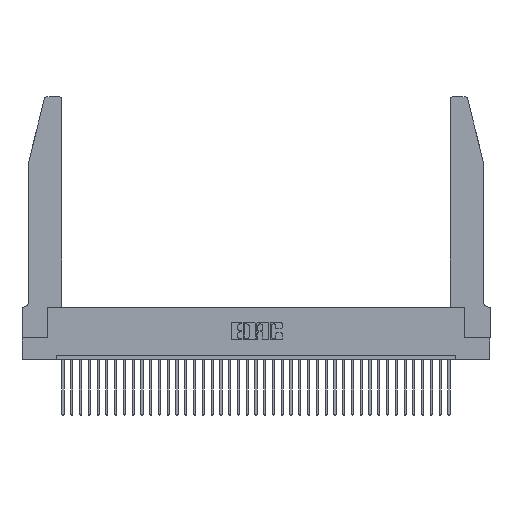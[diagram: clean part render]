
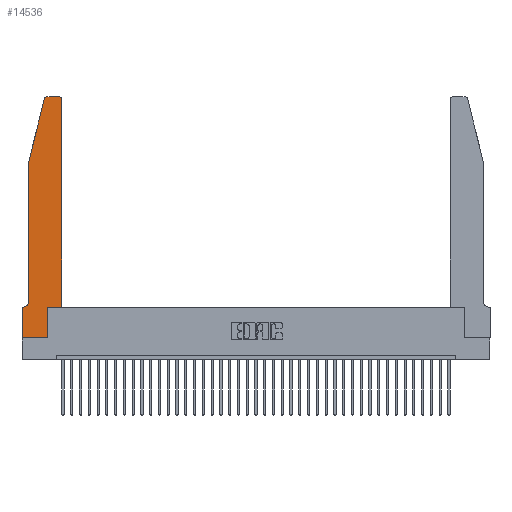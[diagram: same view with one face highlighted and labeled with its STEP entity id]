
A CAD part, top view. The second image highlights one B-rep face of the part: STEP entity #14536.
In plain terms, the highlighted planar face has unit normal (0, 0, 1).
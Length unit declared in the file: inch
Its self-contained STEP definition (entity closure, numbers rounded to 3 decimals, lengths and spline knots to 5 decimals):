
#27 = ORIENTED_EDGE ( 'NONE', *, *, #2586, .T. ) ;
#439 = VERTEX_POINT ( 'NONE', #1338 ) ;
#661 = LINE ( 'NONE', #3811, #19276 ) ;
#669 = DIRECTION ( 'NONE',  ( 1., 0., 0. ) ) ;
#900 = ORIENTED_EDGE ( 'NONE', *, *, #21113, .T. ) ;
#1338 = CARTESIAN_POINT ( 'NONE',  ( 0.284, 2.75, 0.37 ) ) ;
#1552 = ORIENTED_EDGE ( 'NONE', *, *, #27397, .T. ) ;
#1887 = EDGE_CURVE ( 'NONE', #439, #12241, #6059, .T. ) ;
#2379 = DIRECTION ( 'NONE',  ( 1., 0., 0. ) ) ;
#2560 = VECTOR ( 'NONE', #28213, 39.37008 ) ;
#2586 = EDGE_CURVE ( 'NONE', #36108, #38092, #12020, .T. ) ;
#3017 = VECTOR ( 'NONE', #18549, 39.37008 ) ;
#3510 = ORIENTED_EDGE ( 'NONE', *, *, #21230, .T. ) ;
#3811 = CARTESIAN_POINT ( 'NONE',  ( 0.4505, 0.35, 0.37 ) ) ;
#4229 = DIRECTION ( 'NONE',  ( 0., -1., 0. ) ) ;
#4779 = CARTESIAN_POINT ( 'NONE',  ( 0., 0., 0.37 ) ) ;
#5054 = EDGE_CURVE ( 'NONE', #34523, #29858, #28505, .T. ) ;
#5510 = ORIENTED_EDGE ( 'NONE', *, *, #1887, .T. ) ;
#5737 = AXIS2_PLACEMENT_3D ( 'NONE', #20176, #38187, #2379 ) ;
#6059 = CIRCLE ( 'NONE', #23734, 0.03 ) ;
#6808 = CARTESIAN_POINT ( 'NONE',  ( 0.4505, 0.35, 0.37 ) ) ;
#7506 = CARTESIAN_POINT ( 'NONE',  ( 0.4505, 2.72, 0.37 ) ) ;
#7575 = EDGE_CURVE ( 'NONE', #21696, #34523, #20828, .T. ) ;
#7749 = CARTESIAN_POINT ( 'NONE',  ( 0.4505, 0.35, 0.37 ) ) ;
#7900 = DIRECTION ( 'NONE',  ( 1., 0., 0. ) ) ;
#7916 = VERTEX_POINT ( 'NONE', #7506 ) ;
#8160 = DIRECTION ( 'NONE',  ( 1., 0., 0. ) ) ;
#8481 = CARTESIAN_POINT ( 'NONE',  ( 0.0055, 0.35, 0.37 ) ) ;
#9003 = DIRECTION ( 'NONE',  ( 0., 0., 1. ) ) ;
#9272 = LINE ( 'NONE', #36241, #23225 ) ;
#9923 = EDGE_CURVE ( 'NONE', #19234, #21696, #10571, .T. ) ;
#9963 = ORIENTED_EDGE ( 'NONE', *, *, #11675, .T. ) ;
#10032 = CARTESIAN_POINT ( 'NONE',  ( 0.2865, 0., 0.37 ) ) ;
#10311 = AXIS2_PLACEMENT_3D ( 'NONE', #26626, #9003, #669 ) ;
#10571 = LINE ( 'NONE', #36895, #30938 ) ;
#10976 = VERTEX_POINT ( 'NONE', #34652 ) ;
#11675 = EDGE_CURVE ( 'NONE', #7916, #10976, #25784, .T. ) ;
#11745 = VECTOR ( 'NONE', #31426, 39.37008 ) ;
#11916 = EDGE_CURVE ( 'NONE', #13918, #7916, #661, .T. ) ;
#12020 = LINE ( 'NONE', #12083, #21261 ) ;
#12083 = CARTESIAN_POINT ( 'NONE',  ( 0.2865, 0.35, 0.37 ) ) ;
#12241 = VERTEX_POINT ( 'NONE', #16559 ) ;
#12254 = LINE ( 'NONE', #35901, #3017 ) ;
#12958 = CARTESIAN_POINT ( 'NONE',  ( 0.2865, 0.35, 0.37 ) ) ;
#13741 = CARTESIAN_POINT ( 'NONE',  ( 0., 0., 0.37 ) ) ;
#13918 = VERTEX_POINT ( 'NONE', #6808 ) ;
#13944 = CARTESIAN_POINT ( 'NONE',  ( 0.0055, 0.42, 0.37 ) ) ;
#14076 = DIRECTION ( 'NONE',  ( 0., 0., -1. ) ) ;
#14536 = ADVANCED_FACE ( 'NONE', ( #22300 ), #17687, .T. ) ;
#14824 = EDGE_CURVE ( 'NONE', #10976, #439, #9272, .T. ) ;
#14946 = CARTESIAN_POINT ( 'NONE',  ( 0.284, 2.72, 0.37 ) ) ;
#15090 = DIRECTION ( 'NONE',  ( 0., 1., 0. ) ) ;
#16528 = ORIENTED_EDGE ( 'NONE', *, *, #7575, .T. ) ;
#16559 = CARTESIAN_POINT ( 'NONE',  ( 0.25487, 2.72718, 0.37 ) ) ;
#17304 = ORIENTED_EDGE ( 'NONE', *, *, #29961, .T. ) ;
#17687 = PLANE ( 'NONE',  #10311 ) ;
#18549 = DIRECTION ( 'NONE',  ( -0.239, -0.971, 0. ) ) ;
#19234 = VERTEX_POINT ( 'NONE', #24349 ) ;
#19276 = VECTOR ( 'NONE', #30880, 39.37008 ) ;
#20176 = CARTESIAN_POINT ( 'NONE',  ( 0.4205, 2.72, 0.37 ) ) ;
#20180 = VERTEX_POINT ( 'NONE', #24762 ) ;
#20828 = CIRCLE ( 'NONE', #27363, 0.07 ) ;
#21113 = EDGE_CURVE ( 'NONE', #20180, #36108, #26220, .T. ) ;
#21230 = EDGE_CURVE ( 'NONE', #12241, #19234, #12254, .T. ) ;
#21261 = VECTOR ( 'NONE', #15090, 39.37008 ) ;
#21696 = VERTEX_POINT ( 'NONE', #31129 ) ;
#22029 = LINE ( 'NONE', #7749, #2560 ) ;
#22300 = FACE_OUTER_BOUND ( 'NONE', #22738, .T. ) ;
#22738 = EDGE_LOOP ( 'NONE', ( #34555, #5510, #3510, #27097, #16528, #27089, #1552, #900, #27, #17304, #29518, #9963 ) ) ;
#23225 = VECTOR ( 'NONE', #33301, 39.37008 ) ;
#23734 = AXIS2_PLACEMENT_3D ( 'NONE', #14946, #23976, #8160 ) ;
#23976 = DIRECTION ( 'NONE',  ( 0., 0., 1. ) ) ;
#24349 = CARTESIAN_POINT ( 'NONE',  ( 0.0755, 2., 0.37 ) ) ;
#24762 = CARTESIAN_POINT ( 'NONE',  ( 0., 0., 0.37 ) ) ;
#25153 = DIRECTION ( 'NONE',  ( -1., 0., 0. ) ) ;
#25784 = CIRCLE ( 'NONE', #5737, 0.03 ) ;
#26220 = LINE ( 'NONE', #13741, #32194 ) ;
#26626 = CARTESIAN_POINT ( 'NONE',  ( 0., 0.35, 0.37 ) ) ;
#27050 = CARTESIAN_POINT ( 'NONE',  ( 0.0755, 0.35, 0.37 ) ) ;
#27089 = ORIENTED_EDGE ( 'NONE', *, *, #5054, .T. ) ;
#27097 = ORIENTED_EDGE ( 'NONE', *, *, #9923, .T. ) ;
#27363 = AXIS2_PLACEMENT_3D ( 'NONE', #13944, #14076, #32129 ) ;
#27397 = EDGE_CURVE ( 'NONE', #29858, #20180, #35291, .T. ) ;
#28213 = DIRECTION ( 'NONE',  ( 1., 0., 0. ) ) ;
#28474 = CARTESIAN_POINT ( 'NONE',  ( 0., 0.35, 0.37 ) ) ;
#28505 = LINE ( 'NONE', #27050, #29391 ) ;
#29391 = VECTOR ( 'NONE', #25153, 39.37008 ) ;
#29518 = ORIENTED_EDGE ( 'NONE', *, *, #11916, .T. ) ;
#29858 = VERTEX_POINT ( 'NONE', #28474 ) ;
#29961 = EDGE_CURVE ( 'NONE', #38092, #13918, #22029, .T. ) ;
#30880 = DIRECTION ( 'NONE',  ( 0., 1., 0. ) ) ;
#30938 = VECTOR ( 'NONE', #4229, 39.37008 ) ;
#31129 = CARTESIAN_POINT ( 'NONE',  ( 0.0755, 0.42, 0.37 ) ) ;
#31426 = DIRECTION ( 'NONE',  ( 0., -1., 0. ) ) ;
#32129 = DIRECTION ( 'NONE',  ( -1., 0., 0. ) ) ;
#32194 = VECTOR ( 'NONE', #7900, 39.37008 ) ;
#33301 = DIRECTION ( 'NONE',  ( -1., 0., 0. ) ) ;
#34523 = VERTEX_POINT ( 'NONE', #8481 ) ;
#34555 = ORIENTED_EDGE ( 'NONE', *, *, #14824, .T. ) ;
#34652 = CARTESIAN_POINT ( 'NONE',  ( 0.4205, 2.75, 0.37 ) ) ;
#35291 = LINE ( 'NONE', #4779, #11745 ) ;
#35901 = CARTESIAN_POINT ( 'NONE',  ( 0.0755, 2., 0.37 ) ) ;
#36108 = VERTEX_POINT ( 'NONE', #10032 ) ;
#36241 = CARTESIAN_POINT ( 'NONE',  ( 0.2605, 2.75, 0.37 ) ) ;
#36895 = CARTESIAN_POINT ( 'NONE',  ( 0.0755, 2., 0.37 ) ) ;
#38092 = VERTEX_POINT ( 'NONE', #12958 ) ;
#38187 = DIRECTION ( 'NONE',  ( 0., 0., 1. ) ) ;
